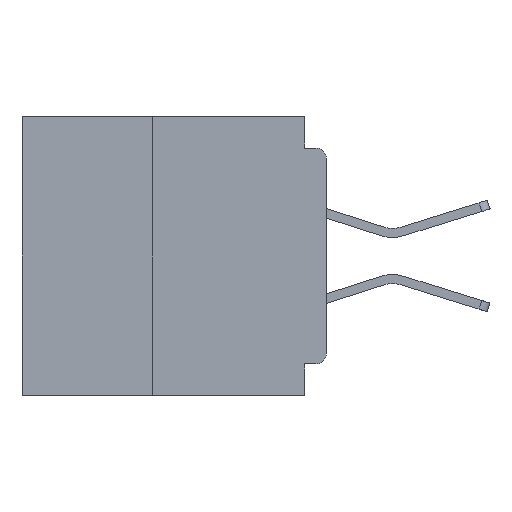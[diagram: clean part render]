
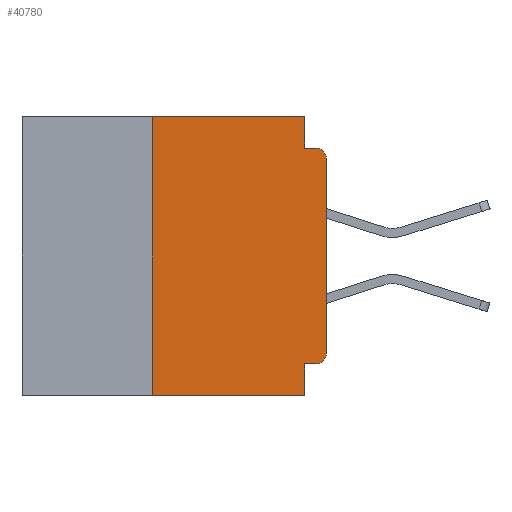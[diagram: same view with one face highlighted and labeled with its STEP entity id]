
A CAD part, left-side view. The second image highlights one B-rep face of the part: STEP entity #40780.
In plain terms, the highlighted planar face has unit normal (-1, 0, 0).
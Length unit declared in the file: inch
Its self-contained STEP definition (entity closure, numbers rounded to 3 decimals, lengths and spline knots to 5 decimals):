
#645 = VERTEX_POINT ( 'NONE', #30381 ) ;
#813 = ORIENTED_EDGE ( 'NONE', *, *, #7143, .T. ) ;
#1229 = VECTOR ( 'NONE', #28995, 39.37008 ) ;
#1994 = EDGE_CURVE ( 'NONE', #2113, #23728, #23118, .T. ) ;
#2113 = VERTEX_POINT ( 'NONE', #23337 ) ;
#2238 = FACE_OUTER_BOUND ( 'NONE', #27551, .T. ) ;
#2941 = ORIENTED_EDGE ( 'NONE', *, *, #40720, .T. ) ;
#3150 = VECTOR ( 'NONE', #10749, 39.37008 ) ;
#3251 = DIRECTION ( 'NONE',  ( -1., 0., 0. ) ) ;
#4475 = CARTESIAN_POINT ( 'NONE',  ( 0., 0.031, -0.4 ) ) ;
#4844 = CARTESIAN_POINT ( 'NONE',  ( 0., 0.437, 0. ) ) ;
#5093 = VERTEX_POINT ( 'NONE', #31976 ) ;
#5346 = DIRECTION ( 'NONE',  ( -1., 0., 0. ) ) ;
#5462 = VECTOR ( 'NONE', #36762, 39.37008 ) ;
#6277 = EDGE_CURVE ( 'NONE', #21735, #23728, #9745, .T. ) ;
#7143 = EDGE_CURVE ( 'NONE', #5093, #7614, #27691, .T. ) ;
#7426 = DIRECTION ( 'NONE',  ( 0., -1., 0. ) ) ;
#7476 = CARTESIAN_POINT ( 'NONE',  ( 0., 0.25, -0.4 ) ) ;
#7614 = VERTEX_POINT ( 'NONE', #19567 ) ;
#7950 = EDGE_CURVE ( 'NONE', #7614, #14165, #40935, .T. ) ;
#8239 = AXIS2_PLACEMENT_3D ( 'NONE', #24534, #5346, #27720 ) ;
#8313 = VECTOR ( 'NONE', #10307, 39.37008 ) ;
#9590 = ORIENTED_EDGE ( 'NONE', *, *, #6277, .T. ) ;
#9745 = LINE ( 'NONE', #32026, #1229 ) ;
#10307 = DIRECTION ( 'NONE',  ( 0., 0., -1. ) ) ;
#10515 = DIRECTION ( 'NONE',  ( 0., 0., 1. ) ) ;
#10585 = EDGE_CURVE ( 'NONE', #21735, #20535, #16077, .T. ) ;
#10749 = DIRECTION ( 'NONE',  ( 0., 0., 1. ) ) ;
#11345 = LINE ( 'NONE', #16670, #8313 ) ;
#12261 = EDGE_CURVE ( 'NONE', #18687, #2113, #26379, .T. ) ;
#12671 = VERTEX_POINT ( 'NONE', #22668 ) ;
#12759 = EDGE_CURVE ( 'NONE', #645, #12671, #11345, .T. ) ;
#12911 = LINE ( 'NONE', #29785, #37279 ) ;
#13306 = ORIENTED_EDGE ( 'NONE', *, *, #12759, .F. ) ;
#13618 = VECTOR ( 'NONE', #29462, 39.37008 ) ;
#14165 = VERTEX_POINT ( 'NONE', #18542 ) ;
#15192 = PLANE ( 'NONE',  #25421 ) ;
#15517 = AXIS2_PLACEMENT_3D ( 'NONE', #22489, #3251, #25694 ) ;
#16077 = LINE ( 'NONE', #26450, #23553 ) ;
#16670 = CARTESIAN_POINT ( 'NONE',  ( 0., 0.031, 0. ) ) ;
#17399 = DIRECTION ( 'NONE',  ( 0., 1., 0. ) ) ;
#18524 = DIRECTION ( 'NONE',  ( 0., 0., -1. ) ) ;
#18542 = CARTESIAN_POINT ( 'NONE',  ( 0., 0.015, -0.045 ) ) ;
#18662 = ORIENTED_EDGE ( 'NONE', *, *, #22615, .F. ) ;
#18687 = VERTEX_POINT ( 'NONE', #26476 ) ;
#19386 = ORIENTED_EDGE ( 'NONE', *, *, #10585, .F. ) ;
#19567 = CARTESIAN_POINT ( 'NONE',  ( 0., 0., -0.06 ) ) ;
#20535 = VERTEX_POINT ( 'NONE', #39583 ) ;
#21735 = VERTEX_POINT ( 'NONE', #7476 ) ;
#22489 = CARTESIAN_POINT ( 'NONE',  ( 0., 0.015, -0.06 ) ) ;
#22615 = EDGE_CURVE ( 'NONE', #20535, #645, #38345, .T. ) ;
#22668 = CARTESIAN_POINT ( 'NONE',  ( 0., 0.031, -0.045 ) ) ;
#23118 = LINE ( 'NONE', #31142, #13618 ) ;
#23337 = CARTESIAN_POINT ( 'NONE',  ( 0., 0.031, -0.355 ) ) ;
#23553 = VECTOR ( 'NONE', #10515, 39.37008 ) ;
#23728 = VERTEX_POINT ( 'NONE', #4475 ) ;
#24534 = CARTESIAN_POINT ( 'NONE',  ( 0., 0.015, -0.34 ) ) ;
#25421 = AXIS2_PLACEMENT_3D ( 'NONE', #27862, #37529, #18524 ) ;
#25694 = DIRECTION ( 'NONE',  ( 0., 0., -1. ) ) ;
#26047 = ORIENTED_EDGE ( 'NONE', *, *, #1994, .F. ) ;
#26379 = LINE ( 'NONE', #36373, #35759 ) ;
#26450 = CARTESIAN_POINT ( 'NONE',  ( 0., 0.25, -0.4 ) ) ;
#26476 = CARTESIAN_POINT ( 'NONE',  ( 0., 0.015, -0.355 ) ) ;
#27502 = ORIENTED_EDGE ( 'NONE', *, *, #33632, .F. ) ;
#27551 = EDGE_LOOP ( 'NONE', ( #813, #34519, #27502, #13306, #18662, #19386, #9590, #26047, #37300, #2941 ) ) ;
#27691 = LINE ( 'NONE', #33080, #3150 ) ;
#27720 = DIRECTION ( 'NONE',  ( 0., 0., -1. ) ) ;
#27862 = CARTESIAN_POINT ( 'NONE',  ( 0., 0.437, 0. ) ) ;
#28995 = DIRECTION ( 'NONE',  ( 0., -1., 0. ) ) ;
#29462 = DIRECTION ( 'NONE',  ( 0., 0., -1. ) ) ;
#29785 = CARTESIAN_POINT ( 'NONE',  ( 0., 0., -0.045 ) ) ;
#30381 = CARTESIAN_POINT ( 'NONE',  ( 0., 0.031, 0. ) ) ;
#30765 = CIRCLE ( 'NONE', #8239, 0.015 ) ;
#31142 = CARTESIAN_POINT ( 'NONE',  ( 0., 0.031, -0.4 ) ) ;
#31976 = CARTESIAN_POINT ( 'NONE',  ( 0., 0., -0.34 ) ) ;
#32026 = CARTESIAN_POINT ( 'NONE',  ( 0., 0.437, -0.4 ) ) ;
#33080 = CARTESIAN_POINT ( 'NONE',  ( 0., 0., 0. ) ) ;
#33632 = EDGE_CURVE ( 'NONE', #12671, #14165, #12911, .T. ) ;
#34519 = ORIENTED_EDGE ( 'NONE', *, *, #7950, .T. ) ;
#35759 = VECTOR ( 'NONE', #17399, 39.37008 ) ;
#36373 = CARTESIAN_POINT ( 'NONE',  ( 0., 0., -0.355 ) ) ;
#36762 = DIRECTION ( 'NONE',  ( 0., -1., 0. ) ) ;
#37279 = VECTOR ( 'NONE', #7426, 39.37008 ) ;
#37300 = ORIENTED_EDGE ( 'NONE', *, *, #12261, .F. ) ;
#37529 = DIRECTION ( 'NONE',  ( 1., 0., 0. ) ) ;
#38345 = LINE ( 'NONE', #4844, #5462 ) ;
#39583 = CARTESIAN_POINT ( 'NONE',  ( 0., 0.25, 0. ) ) ;
#40720 = EDGE_CURVE ( 'NONE', #18687, #5093, #30765, .T. ) ;
#40780 = ADVANCED_FACE ( 'NONE', ( #2238 ), #15192, .F. ) ;
#40935 = CIRCLE ( 'NONE', #15517, 0.015 ) ;
